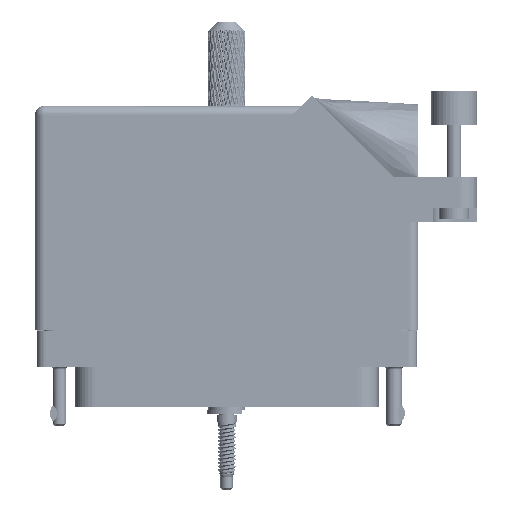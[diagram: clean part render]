
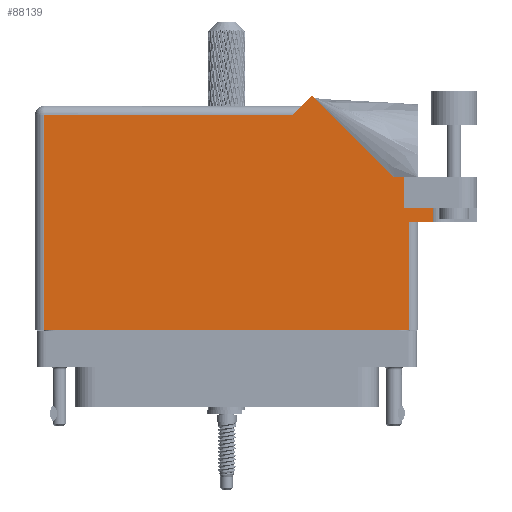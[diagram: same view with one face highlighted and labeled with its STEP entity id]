
A CAD part, front view. The second image highlights one B-rep face of the part: STEP entity #88139.
In plain terms, the highlighted face is planar.
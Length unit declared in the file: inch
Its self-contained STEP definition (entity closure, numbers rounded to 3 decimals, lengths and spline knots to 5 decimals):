
#4461 = CARTESIAN_POINT ( 'NONE',  ( -1.306, 1.43, 0.455 ) ) ;
#6861 = CARTESIAN_POINT ( 'NONE',  ( 1.14042, 0.944, 0.455 ) ) ;
#9483 = ORIENTED_EDGE ( 'NONE', *, *, #29583, .F. ) ;
#12813 = DIRECTION ( 'NONE',  ( -1., 0., 0. ) ) ;
#13773 = EDGE_CURVE ( 'NONE', #23205, #46562, #93019, .T. ) ;
#13967 = CARTESIAN_POINT ( 'NONE',  ( 0.513, 1.43, 0.455 ) ) ;
#14091 = VECTOR ( 'NONE', #102764, 39.37008 ) ;
#15942 = VERTEX_POINT ( 'NONE', #87533 ) ;
#16052 = LINE ( 'NONE', #40305, #123515 ) ;
#16589 = CARTESIAN_POINT ( 'NONE',  ( 0.58371, 1.50071, 0.455 ) ) ;
#18007 = DIRECTION ( 'NONE',  ( 0., -1., 0. ) ) ;
#19348 = EDGE_CURVE ( 'NONE', #101978, #15942, #16052, .T. ) ;
#19631 = DIRECTION ( 'NONE',  ( 1., 0., 0. ) ) ;
#19723 = CARTESIAN_POINT ( 'NONE',  ( 0.451, 1.368, 0.455 ) ) ;
#22356 = VECTOR ( 'NONE', #19631, 39.37008 ) ;
#23205 = VERTEX_POINT ( 'NONE', #19723 ) ;
#26727 = VECTOR ( 'NONE', #62469, 39.37008 ) ;
#28686 = VECTOR ( 'NONE', #124456, 39.37008 ) ;
#29046 = LINE ( 'NONE', #124220, #82841 ) ;
#29583 = EDGE_CURVE ( 'NONE', #62178, #54705, #93005, .T. ) ;
#32826 = DIRECTION ( 'NONE',  ( -1., 0., 0. ) ) ;
#37526 = ORIENTED_EDGE ( 'NONE', *, *, #103653, .T. ) ;
#37917 = LINE ( 'NONE', #96195, #28686 ) ;
#40305 = CARTESIAN_POINT ( 'NONE',  ( 1.706, 0.944, 0.455 ) ) ;
#45568 = CARTESIAN_POINT ( 'NONE',  ( 1.4075, 0.731, 0.455 ) ) ;
#45717 = DIRECTION ( 'NONE',  ( 0., -1., 0. ) ) ;
#46562 = VERTEX_POINT ( 'NONE', #73357 ) ;
#51193 = CARTESIAN_POINT ( 'NONE',  ( 1.206, 0.944, 0.455 ) ) ;
#53928 = CARTESIAN_POINT ( 'NONE',  ( -1.306, -0.1, 0.455 ) ) ;
#54421 = EDGE_CURVE ( 'NONE', #85571, #110837, #122995, .T. ) ;
#54705 = VERTEX_POINT ( 'NONE', #45568 ) ;
#55761 = EDGE_CURVE ( 'NONE', #110837, #101588, #102871, .T. ) ;
#57290 = CARTESIAN_POINT ( 'NONE',  ( 1.244, 0.637, 0.455 ) ) ;
#57683 = VECTOR ( 'NONE', #71467, 39.37008 ) ;
#57917 = ORIENTED_EDGE ( 'NONE', *, *, #108319, .F. ) ;
#62178 = VERTEX_POINT ( 'NONE', #77924 ) ;
#62469 = DIRECTION ( 'NONE',  ( -0.707, -0.707, 0. ) ) ;
#63280 = PLANE ( 'NONE',  #120567 ) ;
#63612 = CARTESIAN_POINT ( 'NONE',  ( 1.244, -0.1, 0.455 ) ) ;
#64793 = ORIENTED_EDGE ( 'NONE', *, *, #85874, .T. ) ;
#66116 = EDGE_CURVE ( 'NONE', #101588, #125632, #77552, .T. ) ;
#70223 = CARTESIAN_POINT ( 'NONE',  ( 1.4075, 0.637, 0.455 ) ) ;
#71333 = VERTEX_POINT ( 'NONE', #16589 ) ;
#71467 = DIRECTION ( 'NONE',  ( 1., 0., 0. ) ) ;
#73357 = CARTESIAN_POINT ( 'NONE',  ( -1.244, 1.368, 0.455 ) ) ;
#74114 = CARTESIAN_POINT ( 'NONE',  ( 1.244, 0.637, 0.455 ) ) ;
#76768 = CARTESIAN_POINT ( 'NONE',  ( 1.4075, 1.06177, 0.455 ) ) ;
#77552 = LINE ( 'NONE', #119498, #57683 ) ;
#77924 = CARTESIAN_POINT ( 'NONE',  ( 1.206, 0.731, 0.455 ) ) ;
#78378 = CARTESIAN_POINT ( 'NONE',  ( 1.206, 0.731, 0.455 ) ) ;
#78875 = ORIENTED_EDGE ( 'NONE', *, *, #125750, .T. ) ;
#80615 = CARTESIAN_POINT ( 'NONE',  ( -1.306, 1.368, 0.455 ) ) ;
#80781 = CARTESIAN_POINT ( 'NONE',  ( -1.244, -0.1, 0.455 ) ) ;
#81758 = EDGE_CURVE ( 'NONE', #71333, #23205, #108019, .T. ) ;
#81772 = DIRECTION ( 'NONE',  ( 0., 0., -1. ) ) ;
#82841 = VECTOR ( 'NONE', #45717, 39.37008 ) ;
#84704 = DIRECTION ( 'NONE',  ( 0., 1., 0. ) ) ;
#85571 = VERTEX_POINT ( 'NONE', #80781 ) ;
#85874 = EDGE_CURVE ( 'NONE', #15942, #71333, #95471, .T. ) ;
#87533 = CARTESIAN_POINT ( 'NONE',  ( 1.14042, 0.944, 0.455 ) ) ;
#88139 = ADVANCED_FACE ( 'NONE', ( #126072 ), #63280, .F. ) ;
#88180 = ORIENTED_EDGE ( 'NONE', *, *, #55761, .T. ) ;
#89069 = VECTOR ( 'NONE', #124427, 39.37008 ) ;
#91966 = ORIENTED_EDGE ( 'NONE', *, *, #66116, .T. ) ;
#93005 = LINE ( 'NONE', #78378, #22356 ) ;
#93019 = LINE ( 'NONE', #80615, #115924 ) ;
#94101 = VECTOR ( 'NONE', #18007, 39.37008 ) ;
#95471 = LINE ( 'NONE', #6861, #89069 ) ;
#96195 = CARTESIAN_POINT ( 'NONE',  ( 1.206, 0.731, 0.455 ) ) ;
#99168 = ORIENTED_EDGE ( 'NONE', *, *, #19348, .T. ) ;
#99868 = VECTOR ( 'NONE', #84704, 39.37008 ) ;
#101588 = VERTEX_POINT ( 'NONE', #74114 ) ;
#101978 = VERTEX_POINT ( 'NONE', #51193 ) ;
#102764 = DIRECTION ( 'NONE',  ( 1., 0., 0. ) ) ;
#102871 = LINE ( 'NONE', #57290, #99868 ) ;
#103653 = EDGE_CURVE ( 'NONE', #62178, #101978, #37917, .T. ) ;
#104727 = LINE ( 'NONE', #76768, #94101 ) ;
#108019 = LINE ( 'NONE', #13967, #26727 ) ;
#108178 = ORIENTED_EDGE ( 'NONE', *, *, #54421, .T. ) ;
#108319 = EDGE_CURVE ( 'NONE', #54705, #125632, #104727, .T. ) ;
#110837 = VERTEX_POINT ( 'NONE', #63612 ) ;
#115924 = VECTOR ( 'NONE', #12813, 39.37008 ) ;
#116903 = EDGE_LOOP ( 'NONE', ( #108178, #88180, #91966, #57917, #9483, #37526, #99168, #64793, #118662, #117128, #78875 ) ) ;
#117128 = ORIENTED_EDGE ( 'NONE', *, *, #13773, .T. ) ;
#118662 = ORIENTED_EDGE ( 'NONE', *, *, #81758, .T. ) ;
#119498 = CARTESIAN_POINT ( 'NONE',  ( 1.306, 0.637, 0.455 ) ) ;
#119623 = DIRECTION ( 'NONE',  ( -1., 0., 0. ) ) ;
#120567 = AXIS2_PLACEMENT_3D ( 'NONE', #4461, #81772, #32826 ) ;
#122995 = LINE ( 'NONE', #53928, #14091 ) ;
#123515 = VECTOR ( 'NONE', #119623, 39.37008 ) ;
#124220 = CARTESIAN_POINT ( 'NONE',  ( -1.244, -0.1, 0.455 ) ) ;
#124427 = DIRECTION ( 'NONE',  ( -0.707, 0.707, 0. ) ) ;
#124456 = DIRECTION ( 'NONE',  ( 0., 1., 0. ) ) ;
#125632 = VERTEX_POINT ( 'NONE', #70223 ) ;
#125750 = EDGE_CURVE ( 'NONE', #46562, #85571, #29046, .T. ) ;
#126072 = FACE_OUTER_BOUND ( 'NONE', #116903, .T. ) ;
